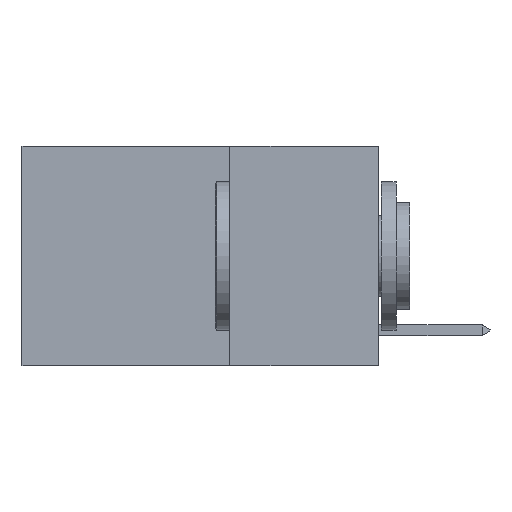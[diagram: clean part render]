
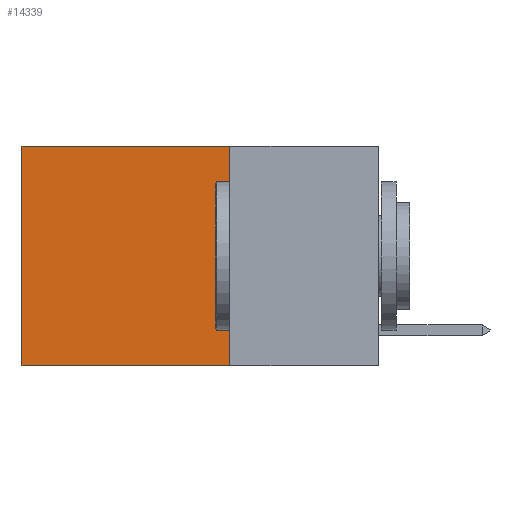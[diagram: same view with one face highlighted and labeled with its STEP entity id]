
A CAD part, left-side view. The second image highlights one B-rep face of the part: STEP entity #14339.
In plain terms, the highlighted planar face has unit normal (-1, 0, 0).
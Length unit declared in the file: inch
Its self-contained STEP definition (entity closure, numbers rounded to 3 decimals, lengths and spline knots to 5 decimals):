
#225 = LINE ( 'NONE', #21847, #18231 ) ;
#1519 = EDGE_CURVE ( 'NONE', #12316, #8957, #2787, .T. ) ;
#1933 = ORIENTED_EDGE ( 'NONE', *, *, #14610, .T. ) ;
#2325 = CARTESIAN_POINT ( 'NONE',  ( 0.2625, 0.25, 0. ) ) ;
#2787 = LINE ( 'NONE', #5162, #15578 ) ;
#3924 = PLANE ( 'NONE',  #17394 ) ;
#5162 = CARTESIAN_POINT ( 'NONE',  ( 0.2625, 0.25, 0. ) ) ;
#5278 = DIRECTION ( 'NONE',  ( 0., 0., -1. ) ) ;
#5305 = FACE_OUTER_BOUND ( 'NONE', #22182, .T. ) ;
#5540 = LINE ( 'NONE', #2325, #14206 ) ;
#5701 = DIRECTION ( 'NONE',  ( 0., 0., -1. ) ) ;
#6337 = DIRECTION ( 'NONE',  ( 0., 1., 0. ) ) ;
#7388 = CARTESIAN_POINT ( 'NONE',  ( 0.2625, 0.25, 0. ) ) ;
#7484 = CARTESIAN_POINT ( 'NONE',  ( 0.2625, 0.6, 0. ) ) ;
#8957 = VERTEX_POINT ( 'NONE', #19046 ) ;
#9917 = DIRECTION ( 'NONE',  ( 0., 0., -1. ) ) ;
#10249 = ORIENTED_EDGE ( 'NONE', *, *, #1519, .F. ) ;
#10306 = EDGE_CURVE ( 'NONE', #8957, #12283, #20783, .T. ) ;
#11512 = CARTESIAN_POINT ( 'NONE',  ( 0.2625, 0.6, -0.37 ) ) ;
#12283 = VERTEX_POINT ( 'NONE', #11512 ) ;
#12293 = VECTOR ( 'NONE', #6337, 39.37008 ) ;
#12316 = VERTEX_POINT ( 'NONE', #20057 ) ;
#14206 = VECTOR ( 'NONE', #17951, 39.37008 ) ;
#14339 = ADVANCED_FACE ( 'NONE', ( #5305 ), #3924, .F. ) ;
#14610 = EDGE_CURVE ( 'NONE', #18145, #12283, #225, .T. ) ;
#15020 = EDGE_CURVE ( 'NONE', #12316, #18145, #5540, .T. ) ;
#15466 = ORIENTED_EDGE ( 'NONE', *, *, #10306, .F. ) ;
#15578 = VECTOR ( 'NONE', #5278, 39.37008 ) ;
#16053 = DIRECTION ( 'NONE',  ( 1., 0., 0. ) ) ;
#16328 = ORIENTED_EDGE ( 'NONE', *, *, #15020, .T. ) ;
#17394 = AXIS2_PLACEMENT_3D ( 'NONE', #7388, #16053, #5701 ) ;
#17951 = DIRECTION ( 'NONE',  ( 0., 1., 0. ) ) ;
#18145 = VERTEX_POINT ( 'NONE', #7484 ) ;
#18231 = VECTOR ( 'NONE', #9917, 39.37008 ) ;
#19046 = CARTESIAN_POINT ( 'NONE',  ( 0.2625, 0.25, -0.37 ) ) ;
#19680 = CARTESIAN_POINT ( 'NONE',  ( 0.2625, 0.25, -0.37 ) ) ;
#20057 = CARTESIAN_POINT ( 'NONE',  ( 0.2625, 0.25, 0. ) ) ;
#20783 = LINE ( 'NONE', #19680, #12293 ) ;
#21847 = CARTESIAN_POINT ( 'NONE',  ( 0.2625, 0.6, 0. ) ) ;
#22182 = EDGE_LOOP ( 'NONE', ( #1933, #15466, #10249, #16328 ) ) ;
